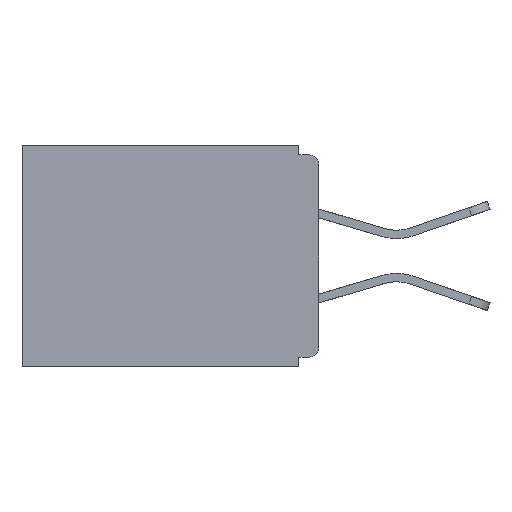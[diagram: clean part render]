
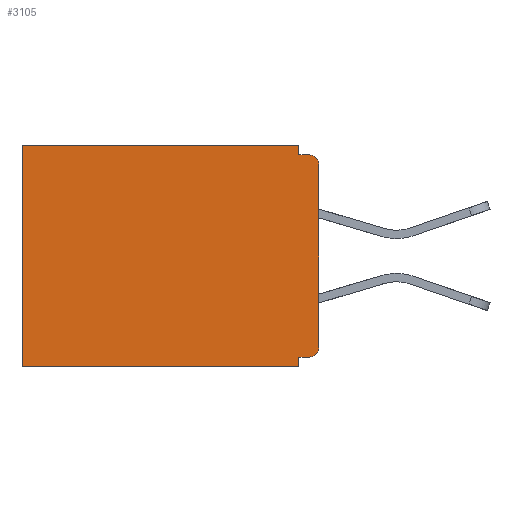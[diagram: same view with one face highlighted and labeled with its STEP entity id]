
A CAD part, left-side view. The second image highlights one B-rep face of the part: STEP entity #3105.
In plain terms, the highlighted planar face has unit normal (-1, 0, 0).
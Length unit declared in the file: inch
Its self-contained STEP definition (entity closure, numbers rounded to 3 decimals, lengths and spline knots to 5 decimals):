
#28 = VERTEX_POINT ( 'NONE', #6537 ) ;
#509 = CARTESIAN_POINT ( 'NONE',  ( 0.298, 0., 0. ) ) ;
#563 = VERTEX_POINT ( 'NONE', #13668 ) ;
#566 = EDGE_CURVE ( 'NONE', #13590, #4670, #12736, .T. ) ;
#873 = CARTESIAN_POINT ( 'NONE',  ( 0.298, 0.031, -0.343 ) ) ;
#1190 = VECTOR ( 'NONE', #5224, 39.37008 ) ;
#1403 = AXIS2_PLACEMENT_3D ( 'NONE', #11866, #9583, #12798 ) ;
#1684 = CARTESIAN_POINT ( 'NONE',  ( 0.298, 0.46, 0. ) ) ;
#1745 = EDGE_CURVE ( 'NONE', #13590, #9829, #10930, .T. ) ;
#1878 = VECTOR ( 'NONE', #2531, 39.37008 ) ;
#1935 = ORIENTED_EDGE ( 'NONE', *, *, #6049, .F. ) ;
#2209 = ORIENTED_EDGE ( 'NONE', *, *, #10723, .T. ) ;
#2283 = LINE ( 'NONE', #6084, #9442 ) ;
#2381 = DIRECTION ( 'NONE',  ( 0., 1., 0. ) ) ;
#2479 = CARTESIAN_POINT ( 'NONE',  ( 0.298, 0.031, -0.343 ) ) ;
#2499 = VECTOR ( 'NONE', #4943, 39.37008 ) ;
#2531 = DIRECTION ( 'NONE',  ( 0., 0., -1. ) ) ;
#3105 = ADVANCED_FACE ( 'NONE', ( #4787 ), #12510, .F. ) ;
#3610 = CARTESIAN_POINT ( 'NONE',  ( 0.298, 0.015, -0.328 ) ) ;
#3799 = CARTESIAN_POINT ( 'NONE',  ( 0.298, 0., -0.328 ) ) ;
#3866 = CARTESIAN_POINT ( 'NONE',  ( 0.298, 0., 0. ) ) ;
#4088 = ORIENTED_EDGE ( 'NONE', *, *, #13307, .F. ) ;
#4318 = DIRECTION ( 'NONE',  ( 0., -1., 0. ) ) ;
#4542 = DIRECTION ( 'NONE',  ( 0., 0., -1. ) ) ;
#4670 = VERTEX_POINT ( 'NONE', #6572 ) ;
#4787 = FACE_OUTER_BOUND ( 'NONE', #5365, .T. ) ;
#4943 = DIRECTION ( 'NONE',  ( 0., 1., 0. ) ) ;
#4999 = AXIS2_PLACEMENT_3D ( 'NONE', #509, #10301, #9215 ) ;
#5224 = DIRECTION ( 'NONE',  ( 0., 0., -1. ) ) ;
#5344 = CARTESIAN_POINT ( 'NONE',  ( 0.298, 0.46, 0. ) ) ;
#5365 = EDGE_LOOP ( 'NONE', ( #9979, #7846, #4088, #6267, #2209, #14108, #11669, #13952, #8866, #1935 ) ) ;
#5442 = EDGE_CURVE ( 'NONE', #9643, #7768, #11825, .T. ) ;
#5569 = VECTOR ( 'NONE', #13523, 39.37008 ) ;
#5827 = LINE ( 'NONE', #2479, #1878 ) ;
#6049 = EDGE_CURVE ( 'NONE', #8524, #9829, #13873, .T. ) ;
#6084 = CARTESIAN_POINT ( 'NONE',  ( 0.298, 0., -0.015 ) ) ;
#6267 = ORIENTED_EDGE ( 'NONE', *, *, #6566, .T. ) ;
#6532 = CARTESIAN_POINT ( 'NONE',  ( 0.298, 0.031, 0. ) ) ;
#6537 = CARTESIAN_POINT ( 'NONE',  ( 0.298, 0.015, -0.015 ) ) ;
#6566 = EDGE_CURVE ( 'NONE', #11327, #13032, #8926, .T. ) ;
#6572 = CARTESIAN_POINT ( 'NONE',  ( 0.298, 0.031, -0.328 ) ) ;
#6584 = EDGE_CURVE ( 'NONE', #8524, #28, #14016, .T. ) ;
#6664 = CARTESIAN_POINT ( 'NONE',  ( 0.298, 0.031, -0.343 ) ) ;
#7768 = VERTEX_POINT ( 'NONE', #7918 ) ;
#7846 = ORIENTED_EDGE ( 'NONE', *, *, #9740, .F. ) ;
#7918 = CARTESIAN_POINT ( 'NONE',  ( 0.298, 0.46, -0.343 ) ) ;
#8113 = AXIS2_PLACEMENT_3D ( 'NONE', #11039, #9933, #4542 ) ;
#8524 = VERTEX_POINT ( 'NONE', #8526 ) ;
#8526 = CARTESIAN_POINT ( 'NONE',  ( 0.298, 0., -0.03 ) ) ;
#8866 = ORIENTED_EDGE ( 'NONE', *, *, #1745, .T. ) ;
#8926 = LINE ( 'NONE', #10031, #9934 ) ;
#9061 = CARTESIAN_POINT ( 'NONE',  ( 0.298, 0., -0.313 ) ) ;
#9177 = DIRECTION ( 'NONE',  ( 0., 0., -1. ) ) ;
#9215 = DIRECTION ( 'NONE',  ( 0., 0., -1. ) ) ;
#9442 = VECTOR ( 'NONE', #4318, 39.37008 ) ;
#9583 = DIRECTION ( 'NONE',  ( -1., 0., 0. ) ) ;
#9643 = VERTEX_POINT ( 'NONE', #6664 ) ;
#9740 = EDGE_CURVE ( 'NONE', #563, #28, #2283, .T. ) ;
#9829 = VERTEX_POINT ( 'NONE', #9061 ) ;
#9933 = DIRECTION ( 'NONE',  ( -1., 0., 0. ) ) ;
#9934 = VECTOR ( 'NONE', #2381, 39.37008 ) ;
#9979 = ORIENTED_EDGE ( 'NONE', *, *, #6584, .T. ) ;
#10031 = CARTESIAN_POINT ( 'NONE',  ( 0.298, 0., 0. ) ) ;
#10301 = DIRECTION ( 'NONE',  ( 1., 0., 0. ) ) ;
#10626 = DIRECTION ( 'NONE',  ( 0., 0., -1. ) ) ;
#10634 = VECTOR ( 'NONE', #9177, 39.37008 ) ;
#10723 = EDGE_CURVE ( 'NONE', #13032, #7768, #11973, .T. ) ;
#10930 = CIRCLE ( 'NONE', #1403, 0.015 ) ;
#11039 = CARTESIAN_POINT ( 'NONE',  ( 0.298, 0.015, -0.03 ) ) ;
#11141 = CARTESIAN_POINT ( 'NONE',  ( 0.298, 0., -0.343 ) ) ;
#11327 = VERTEX_POINT ( 'NONE', #6532 ) ;
#11669 = ORIENTED_EDGE ( 'NONE', *, *, #13665, .F. ) ;
#11825 = LINE ( 'NONE', #11141, #5569 ) ;
#11866 = CARTESIAN_POINT ( 'NONE',  ( 0.298, 0.015, -0.313 ) ) ;
#11973 = LINE ( 'NONE', #5344, #12498 ) ;
#12458 = LINE ( 'NONE', #873, #1190 ) ;
#12498 = VECTOR ( 'NONE', #10626, 39.37008 ) ;
#12510 = PLANE ( 'NONE',  #4999 ) ;
#12736 = LINE ( 'NONE', #3799, #2499 ) ;
#12798 = DIRECTION ( 'NONE',  ( 0., 0., -1. ) ) ;
#13032 = VERTEX_POINT ( 'NONE', #1684 ) ;
#13307 = EDGE_CURVE ( 'NONE', #11327, #563, #5827, .T. ) ;
#13523 = DIRECTION ( 'NONE',  ( 0., 1., 0. ) ) ;
#13590 = VERTEX_POINT ( 'NONE', #3610 ) ;
#13665 = EDGE_CURVE ( 'NONE', #4670, #9643, #12458, .T. ) ;
#13668 = CARTESIAN_POINT ( 'NONE',  ( 0.298, 0.031, -0.015 ) ) ;
#13873 = LINE ( 'NONE', #3866, #10634 ) ;
#13952 = ORIENTED_EDGE ( 'NONE', *, *, #566, .F. ) ;
#14016 = CIRCLE ( 'NONE', #8113, 0.015 ) ;
#14108 = ORIENTED_EDGE ( 'NONE', *, *, #5442, .F. ) ;
